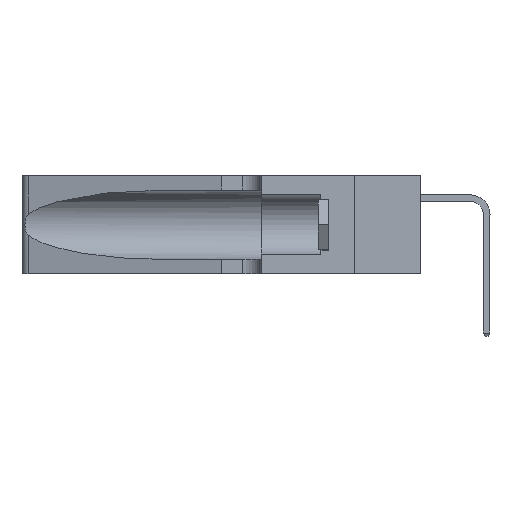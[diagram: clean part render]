
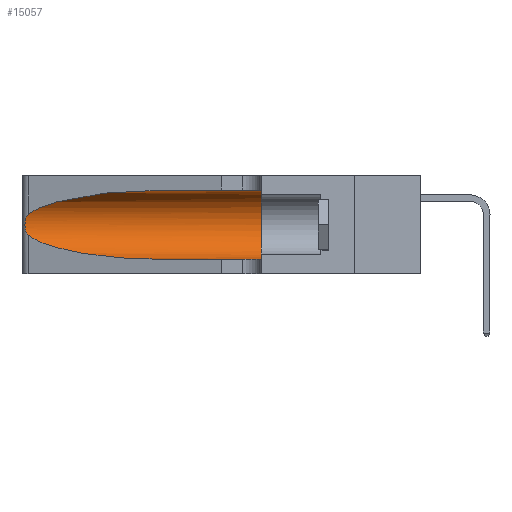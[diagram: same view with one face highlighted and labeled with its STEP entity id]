
A CAD part, left-side view. The second image highlights one B-rep face of the part: STEP entity #15057.
In plain terms, the highlighted cylindrical face has radius 3.308 mm (diameter 6.617 mm), a partial arc.
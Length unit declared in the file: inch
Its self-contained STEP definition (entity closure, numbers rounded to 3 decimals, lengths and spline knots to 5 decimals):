
#1440 = CARTESIAN_POINT ( 'NONE',  ( 0.26018, 1.23835, 0.19895 ) ) ;
#2319 = B_SPLINE_CURVE_WITH_KNOTS ( 'NONE', 3,
 ( #7410, #31009, #16433, #36853, #19388, #1440, #22310, #4483, #25229, #7549, #28167, #10573, #31142, #13544 ),
 .UNSPECIFIED., .F., .F.,
 ( 4, 2, 2, 2, 2, 2, 4 ),
 ( 0., 0.00027, 0.00053, 0.00107, 0.0016, 0.00187, 0.00214 ),
 .UNSPECIFIED. ) ;
#3430 = CARTESIAN_POINT ( 'NONE',  ( 0.1305, 1.61858, 0.05475 ) ) ;
#3519 = DIRECTION ( 'NONE',  ( 0., 1., 0. ) ) ;
#4483 = CARTESIAN_POINT ( 'NONE',  ( 0.26075, 1.23896, 0.178 ) ) ;
#4508 = AXIS2_PLACEMENT_3D ( 'NONE', #35745, #27029, #6342 ) ;
#5109 = EDGE_CURVE ( 'NONE', #11834, #6252, #31613, .T. ) ;
#6173 = AXIS2_PLACEMENT_3D ( 'NONE', #21389, #3519, #24317 ) ;
#6252 = VERTEX_POINT ( 'NONE', #7698 ) ;
#6330 = EDGE_CURVE ( 'NONE', #26088, #25717, #21735, .T. ) ;
#6342 = DIRECTION ( 'NONE',  ( 0., 0., -1. ) ) ;
#7143 = VECTOR ( 'NONE', #24224, 39.37008 ) ;
#7410 = CARTESIAN_POINT ( 'NONE',  ( 0.25487, 1.22718, 0.22369 ) ) ;
#7549 = CARTESIAN_POINT ( 'NONE',  ( 0.25856, 1.23593, 0.16098 ) ) ;
#7698 = CARTESIAN_POINT ( 'NONE',  ( 0.25487, 1.22718, 0.22369 ) ) ;
#7752 = LINE ( 'NONE', #29745, #10572 ) ;
#9180 = CARTESIAN_POINT ( 'NONE',  ( 0.18966, 0.96281, 0.31525 ) ) ;
#10572 = VECTOR ( 'NONE', #12181, 39.37008 ) ;
#10573 = CARTESIAN_POINT ( 'NONE',  ( 0.25639, 1.23186, 0.15144 ) ) ;
#11834 = VERTEX_POINT ( 'NONE', #16210 ) ;
#12181 = DIRECTION ( 'NONE',  ( 0., -1., 0. ) ) ;
#13544 = CARTESIAN_POINT ( 'NONE',  ( 0.25487, 1.22718, 0.14631 ) ) ;
#13554 = ORIENTED_EDGE ( 'NONE', *, *, #5109, .T. ) ;
#14604 = CARTESIAN_POINT ( 'NONE',  ( 0.25487, 1.22718, 0.14631 ) ) ;
#14863 = VERTEX_POINT ( 'NONE', #20314 ) ;
#15057 = ADVANCED_FACE ( 'NONE', ( #33752 ), #25046, .F. ) ;
#16210 = CARTESIAN_POINT ( 'NONE',  ( 0.1305, 0.72297, 0.31525 ) ) ;
#16433 = CARTESIAN_POINT ( 'NONE',  ( 0.25639, 1.23184, 0.21858 ) ) ;
#18625 = ORIENTED_EDGE ( 'NONE', *, *, #35049, .F. ) ;
#19388 = CARTESIAN_POINT ( 'NONE',  ( 0.25854, 1.2359, 0.20912 ) ) ;
#19908 = CARTESIAN_POINT ( 'NONE',  ( 0.2373, 1.15595, 0.08982 ) ) ;
#20314 = CARTESIAN_POINT ( 'NONE',  ( 0.1305, 0.35, 0.31525 ) ) ;
#21389 = CARTESIAN_POINT ( 'NONE',  ( 0.1305, 0.35, 0.185 ) ) ;
#21735 =( BOUNDED_CURVE ( )  B_SPLINE_CURVE ( 3, ( #22816, #19908, #37356, #25747 ),
 .UNSPECIFIED., .F., .F. ) 
 B_SPLINE_CURVE_WITH_KNOTS ( ( 4, 4 ),
 ( 3.44316, 4.71239 ),
 .UNSPECIFIED. ) 
 CURVE ( )  GEOMETRIC_REPRESENTATION_ITEM ( )  RATIONAL_B_SPLINE_CURVE ( ( 1., 0.87, 0.87, 1. ) ) 
 REPRESENTATION_ITEM ( '' )  );
#22310 = CARTESIAN_POINT ( 'NONE',  ( 0.26075, 1.23896, 0.19203 ) ) ;
#22816 = CARTESIAN_POINT ( 'NONE',  ( 0.25487, 1.22718, 0.14631 ) ) ;
#23647 = ORIENTED_EDGE ( 'NONE', *, *, #30644, .T. ) ;
#23873 = CARTESIAN_POINT ( 'NONE',  ( 0.2373, 1.15595, 0.28018 ) ) ;
#24224 = DIRECTION ( 'NONE',  ( 0., -1., 0. ) ) ;
#24317 = DIRECTION ( 'NONE',  ( 0., 0., 1. ) ) ;
#24821 = CARTESIAN_POINT ( 'NONE',  ( 0.1305, 0.35, 0.05475 ) ) ;
#25046 = CYLINDRICAL_SURFACE ( 'NONE', #4508, 0.13025 ) ;
#25229 = CARTESIAN_POINT ( 'NONE',  ( 0.26017, 1.23833, 0.17102 ) ) ;
#25717 = VERTEX_POINT ( 'NONE', #27700 ) ;
#25747 = CARTESIAN_POINT ( 'NONE',  ( 0.1305, 0.72297, 0.05475 ) ) ;
#26088 = VERTEX_POINT ( 'NONE', #14604 ) ;
#26263 = EDGE_LOOP ( 'NONE', ( #13554, #28242, #36418, #23647, #18625, #34159 ) ) ;
#26708 = EDGE_CURVE ( 'NONE', #11834, #14863, #7752, .T. ) ;
#27029 = DIRECTION ( 'NONE',  ( 0., -1., 0. ) ) ;
#27700 = CARTESIAN_POINT ( 'NONE',  ( 0.1305, 0.72297, 0.05475 ) ) ;
#28167 = CARTESIAN_POINT ( 'NONE',  ( 0.25789, 1.23486, 0.15765 ) ) ;
#28242 = ORIENTED_EDGE ( 'NONE', *, *, #34544, .T. ) ;
#29037 = CIRCLE ( 'NONE', #6173, 0.13025 ) ;
#29745 = CARTESIAN_POINT ( 'NONE',  ( 0.1305, 1.61858, 0.31525 ) ) ;
#29749 = CARTESIAN_POINT ( 'NONE',  ( 0.1305, 0.72297, 0.31525 ) ) ;
#29775 = LINE ( 'NONE', #3430, #7143 ) ;
#30644 = EDGE_CURVE ( 'NONE', #25717, #37759, #29775, .T. ) ;
#31009 = CARTESIAN_POINT ( 'NONE',  ( 0.25555, 1.22994, 0.2215 ) ) ;
#31142 = CARTESIAN_POINT ( 'NONE',  ( 0.25555, 1.22993, 0.14849 ) ) ;
#31613 =( BOUNDED_CURVE ( )  B_SPLINE_CURVE ( 3, ( #29749, #9180, #23873, #35625 ),
 .UNSPECIFIED., .F., .T. ) 
 B_SPLINE_CURVE_WITH_KNOTS ( ( 4, 4 ),
 ( 1.5708, 2.84003 ),
 .UNSPECIFIED. ) 
 CURVE ( )  GEOMETRIC_REPRESENTATION_ITEM ( )  RATIONAL_B_SPLINE_CURVE ( ( 1., 0.87, 0.87, 1. ) ) 
 REPRESENTATION_ITEM ( '' )  );
#33752 = FACE_OUTER_BOUND ( 'NONE', #26263, .T. ) ;
#34159 = ORIENTED_EDGE ( 'NONE', *, *, #26708, .F. ) ;
#34544 = EDGE_CURVE ( 'NONE', #6252, #26088, #2319, .T. ) ;
#35049 = EDGE_CURVE ( 'NONE', #14863, #37759, #29037, .T. ) ;
#35625 = CARTESIAN_POINT ( 'NONE',  ( 0.25487, 1.22718, 0.22369 ) ) ;
#35745 = CARTESIAN_POINT ( 'NONE',  ( 0.1305, 1.61858, 0.185 ) ) ;
#36418 = ORIENTED_EDGE ( 'NONE', *, *, #6330, .T. ) ;
#36853 = CARTESIAN_POINT ( 'NONE',  ( 0.25787, 1.23484, 0.2124 ) ) ;
#37356 = CARTESIAN_POINT ( 'NONE',  ( 0.18966, 0.96281, 0.05475 ) ) ;
#37759 = VERTEX_POINT ( 'NONE', #24821 ) ;
